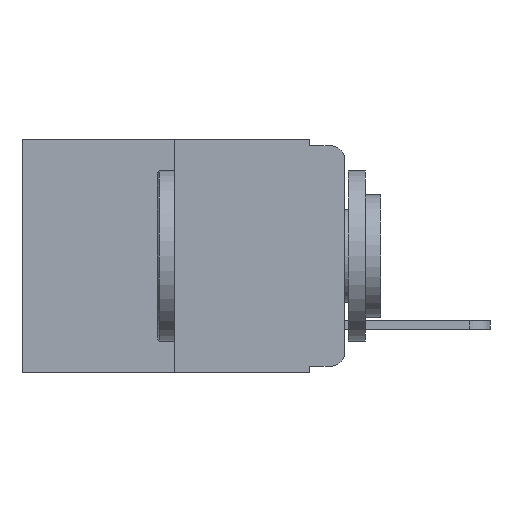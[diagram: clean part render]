
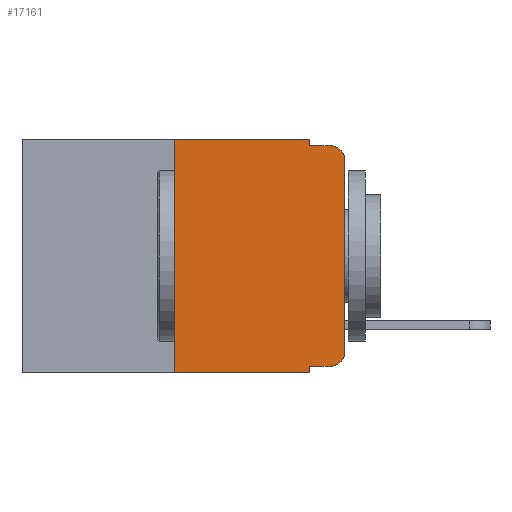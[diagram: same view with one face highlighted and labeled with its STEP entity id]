
A CAD part, left-side view. The second image highlights one B-rep face of the part: STEP entity #17161.
In plain terms, the highlighted planar face has unit normal (-1, 0, 0).
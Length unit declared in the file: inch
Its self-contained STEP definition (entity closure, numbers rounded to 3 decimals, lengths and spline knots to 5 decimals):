
#41 = CARTESIAN_POINT ( 'NONE',  ( 0., 0.051, -0.333 ) ) ;
#64 = CARTESIAN_POINT ( 'NONE',  ( 0., 0.473, 0. ) ) ;
#511 = VERTEX_POINT ( 'NONE', #2297 ) ;
#646 = EDGE_CURVE ( 'NONE', #12363, #4672, #3294, .T. ) ;
#739 = VERTEX_POINT ( 'NONE', #8221 ) ;
#821 = VECTOR ( 'NONE', #13245, 39.37008 ) ;
#1058 = DIRECTION ( 'NONE',  ( 0., 0., -1. ) ) ;
#1300 = VECTOR ( 'NONE', #6208, 39.37008 ) ;
#1738 = CARTESIAN_POINT ( 'NONE',  ( 0., 0.051, -0.01 ) ) ;
#2198 = CARTESIAN_POINT ( 'NONE',  ( 0., 0., -0.03 ) ) ;
#2270 = AXIS2_PLACEMENT_3D ( 'NONE', #64, #14819, #14696 ) ;
#2294 = CARTESIAN_POINT ( 'NONE',  ( 0., 0.02, -0.03 ) ) ;
#2297 = CARTESIAN_POINT ( 'NONE',  ( 0., 0.051, -0.343 ) ) ;
#2319 = DIRECTION ( 'NONE',  ( 0., 0., -1. ) ) ;
#2335 = ORIENTED_EDGE ( 'NONE', *, *, #16026, .T. ) ;
#2426 = CARTESIAN_POINT ( 'NONE',  ( 0., 0.02, -0.313 ) ) ;
#2496 = FACE_OUTER_BOUND ( 'NONE', #3224, .T. ) ;
#2523 = ORIENTED_EDGE ( 'NONE', *, *, #10731, .F. ) ;
#2590 = PLANE ( 'NONE',  #2270 ) ;
#2825 = ORIENTED_EDGE ( 'NONE', *, *, #10228, .T. ) ;
#3224 = EDGE_LOOP ( 'NONE', ( #2335, #14583, #6245, #12267, #4730, #15888, #9691, #2523, #2825, #7826 ) ) ;
#3294 = LINE ( 'NONE', #9295, #821 ) ;
#3405 = VERTEX_POINT ( 'NONE', #6981 ) ;
#4046 = EDGE_CURVE ( 'NONE', #5796, #511, #15155, .T. ) ;
#4642 = VERTEX_POINT ( 'NONE', #41 ) ;
#4672 = VERTEX_POINT ( 'NONE', #12053 ) ;
#4730 = ORIENTED_EDGE ( 'NONE', *, *, #646, .F. ) ;
#4972 = CARTESIAN_POINT ( 'NONE',  ( 0., 0.25, 0. ) ) ;
#5140 = DIRECTION ( 'NONE',  ( -1., 0., 0. ) ) ;
#5178 = EDGE_CURVE ( 'NONE', #13195, #3405, #16137, .T. ) ;
#5475 = CARTESIAN_POINT ( 'NONE',  ( 0., 0.473, -0.343 ) ) ;
#5796 = VERTEX_POINT ( 'NONE', #13793 ) ;
#6127 = DIRECTION ( 'NONE',  ( -1., 0., 0. ) ) ;
#6208 = DIRECTION ( 'NONE',  ( 0., 0., -1. ) ) ;
#6245 = ORIENTED_EDGE ( 'NONE', *, *, #9567, .F. ) ;
#6579 = VECTOR ( 'NONE', #8470, 39.37008 ) ;
#6809 = AXIS2_PLACEMENT_3D ( 'NONE', #2426, #5140, #2319 ) ;
#6861 = LINE ( 'NONE', #8771, #10446 ) ;
#6933 = VERTEX_POINT ( 'NONE', #12592 ) ;
#6981 = CARTESIAN_POINT ( 'NONE',  ( 0., 0., -0.313 ) ) ;
#7505 = CARTESIAN_POINT ( 'NONE',  ( 0., 0.051, 0. ) ) ;
#7629 = EDGE_CURVE ( 'NONE', #16958, #739, #8563, .T. ) ;
#7826 = ORIENTED_EDGE ( 'NONE', *, *, #5178, .T. ) ;
#7874 = CARTESIAN_POINT ( 'NONE',  ( 0., 0., 0. ) ) ;
#8056 = EDGE_CURVE ( 'NONE', #5796, #12363, #6861, .T. ) ;
#8124 = CARTESIAN_POINT ( 'NONE',  ( 0., 0.051, -0.333 ) ) ;
#8221 = CARTESIAN_POINT ( 'NONE',  ( 0., 0.02, -0.01 ) ) ;
#8470 = DIRECTION ( 'NONE',  ( 0., -1., 0. ) ) ;
#8563 = CIRCLE ( 'NONE', #17022, 0.02 ) ;
#8771 = CARTESIAN_POINT ( 'NONE',  ( 0., 0.25, 0. ) ) ;
#9273 = VECTOR ( 'NONE', #14945, 39.37008 ) ;
#9295 = CARTESIAN_POINT ( 'NONE',  ( 0., 0.473, 0. ) ) ;
#9567 = EDGE_CURVE ( 'NONE', #6933, #739, #11849, .T. ) ;
#9691 = ORIENTED_EDGE ( 'NONE', *, *, #4046, .T. ) ;
#9939 = VECTOR ( 'NONE', #15931, 39.37008 ) ;
#10228 = EDGE_CURVE ( 'NONE', #4642, #13195, #16620, .T. ) ;
#10337 = CARTESIAN_POINT ( 'NONE',  ( 0., 0.02, -0.333 ) ) ;
#10446 = VECTOR ( 'NONE', #15325, 39.37008 ) ;
#10731 = EDGE_CURVE ( 'NONE', #4642, #511, #13946, .T. ) ;
#11849 = LINE ( 'NONE', #1738, #6579 ) ;
#12012 = VECTOR ( 'NONE', #16842, 39.37008 ) ;
#12053 = CARTESIAN_POINT ( 'NONE',  ( 0., 0.051, 0. ) ) ;
#12177 = EDGE_CURVE ( 'NONE', #4672, #6933, #12203, .T. ) ;
#12203 = LINE ( 'NONE', #7505, #1300 ) ;
#12267 = ORIENTED_EDGE ( 'NONE', *, *, #12177, .F. ) ;
#12363 = VERTEX_POINT ( 'NONE', #4972 ) ;
#12592 = CARTESIAN_POINT ( 'NONE',  ( 0., 0.051, -0.01 ) ) ;
#13195 = VERTEX_POINT ( 'NONE', #10337 ) ;
#13245 = DIRECTION ( 'NONE',  ( 0., -1., 0. ) ) ;
#13793 = CARTESIAN_POINT ( 'NONE',  ( 0., 0.25, -0.343 ) ) ;
#13946 = LINE ( 'NONE', #14575, #16624 ) ;
#14575 = CARTESIAN_POINT ( 'NONE',  ( 0., 0.051, 0. ) ) ;
#14583 = ORIENTED_EDGE ( 'NONE', *, *, #7629, .T. ) ;
#14696 = DIRECTION ( 'NONE',  ( 0., 0., -1. ) ) ;
#14819 = DIRECTION ( 'NONE',  ( 1., 0., 0. ) ) ;
#14942 = LINE ( 'NONE', #7874, #12012 ) ;
#14945 = DIRECTION ( 'NONE',  ( 0., -1., 0. ) ) ;
#15155 = LINE ( 'NONE', #5475, #9273 ) ;
#15325 = DIRECTION ( 'NONE',  ( 0., 0., 1. ) ) ;
#15888 = ORIENTED_EDGE ( 'NONE', *, *, #8056, .F. ) ;
#15931 = DIRECTION ( 'NONE',  ( 0., -1., 0. ) ) ;
#16026 = EDGE_CURVE ( 'NONE', #3405, #16958, #14942, .T. ) ;
#16137 = CIRCLE ( 'NONE', #6809, 0.02 ) ;
#16620 = LINE ( 'NONE', #8124, #9939 ) ;
#16624 = VECTOR ( 'NONE', #1058, 39.37008 ) ;
#16842 = DIRECTION ( 'NONE',  ( 0., 0., 1. ) ) ;
#16946 = DIRECTION ( 'NONE',  ( 0., 0., -1. ) ) ;
#16958 = VERTEX_POINT ( 'NONE', #2198 ) ;
#17022 = AXIS2_PLACEMENT_3D ( 'NONE', #2294, #6127, #16946 ) ;
#17161 = ADVANCED_FACE ( 'NONE', ( #2496 ), #2590, .F. ) ;
